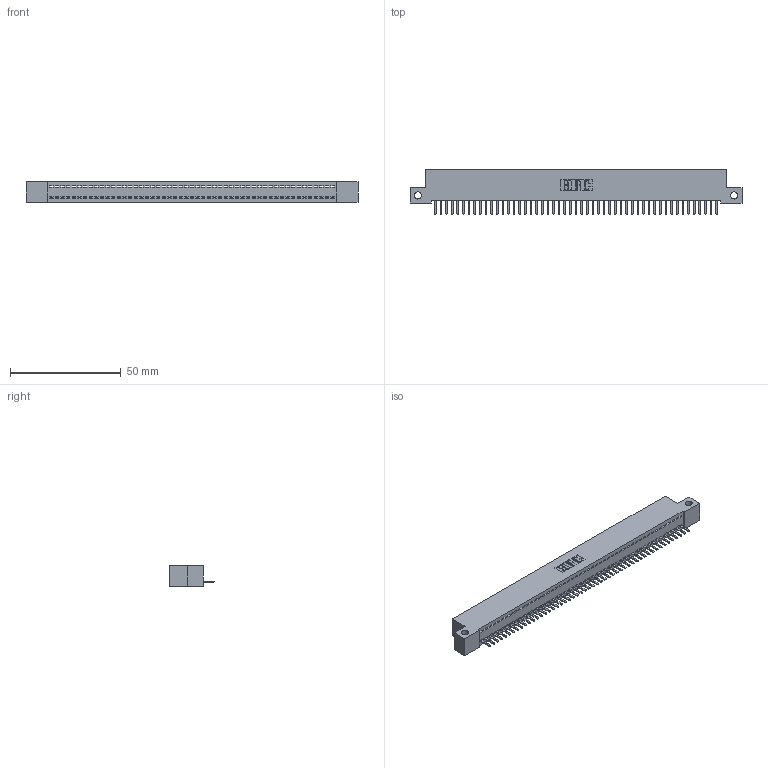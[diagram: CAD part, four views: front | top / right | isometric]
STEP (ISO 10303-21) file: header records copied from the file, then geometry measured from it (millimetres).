
FILE_DESCRIPTION (( 'STEP AP203' ), '1' );
FILE_NAME ('392-051-520-112.STEP', '2019-10-08T11:50:48', ( '' ), ( '' ), 'SwSTEP 2.0', 'SolidWorks 2016', '' );
FILE_SCHEMA (( 'CONFIG_CONTROL_DESIGN' ));
Length unit declared in the file: inch
Products named in the file (3): 342 Part_Side Mount; 345-292-001_345-293-120; 392-051-520-112
Assembly tree (52 placements, depth 2):
  392-051-520-112
    342 Part_Side Mount
    345-292-001_345-293-120  x51
Bounding box: 149.86 x 20.02 x 9.4 mm (x, y, z)
Volume: 12952.2 mm3; surface area: 18555.5 mm2
Topology: 52 solids, 52 shells, 3272 faces, 9683 edges, 6318 vertices
Faces by surface type: plane 2310, cylinder 962
Entity records: 29999 total; most frequent: CARTESIAN_POINT 5191, ORIENTED_EDGE 5166, DIRECTION 4349, EDGE_CURVE 2583, VECTOR 2451, LINE 2451, VERTEX_POINT 1718, AXIS2_PLACEMENT_3D 949
